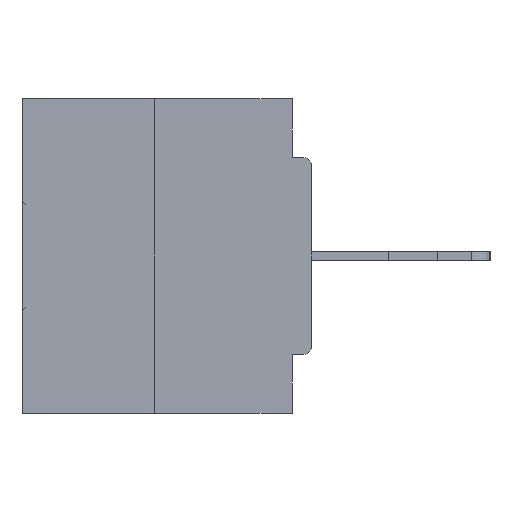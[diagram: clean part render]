
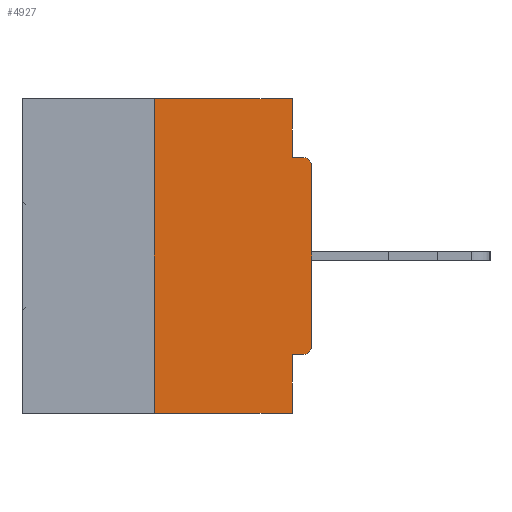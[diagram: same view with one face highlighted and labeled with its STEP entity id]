
A CAD part, left-side view. The second image highlights one B-rep face of the part: STEP entity #4927.
In plain terms, the highlighted planar face has unit normal (-1, 0, 0).
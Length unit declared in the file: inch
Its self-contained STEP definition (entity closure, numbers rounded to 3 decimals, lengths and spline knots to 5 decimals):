
#531 = CARTESIAN_POINT ( 'NONE',  ( 0., 0.031, -0.0935 ) ) ;
#1636 = DIRECTION ( 'NONE',  ( 0., 0., -1. ) ) ;
#2308 = LINE ( 'NONE', #13980, #9226 ) ;
#3226 = CIRCLE ( 'NONE', #31526, 0.015 ) ;
#3934 = EDGE_LOOP ( 'NONE', ( #4821, #33900, #36060, #4055, #22363, #35218, #20865, #37956, #14118, #7076 ) ) ;
#4055 = ORIENTED_EDGE ( 'NONE', *, *, #14420, .F. ) ;
#4821 = ORIENTED_EDGE ( 'NONE', *, *, #16176, .F. ) ;
#4909 = CARTESIAN_POINT ( 'NONE',  ( 0., 0.015, -0.4065 ) ) ;
#4925 = EDGE_CURVE ( 'NONE', #9672, #5532, #18148, .T. ) ;
#4927 = ADVANCED_FACE ( 'NONE', ( #14005 ), #31725, .F. ) ;
#5532 = VERTEX_POINT ( 'NONE', #37963 ) ;
#5896 = DIRECTION ( 'NONE',  ( 0., 1., 0. ) ) ;
#6661 = CARTESIAN_POINT ( 'NONE',  ( 0., 0.031, 0. ) ) ;
#6985 = LINE ( 'NONE', #9278, #9764 ) ;
#7076 = ORIENTED_EDGE ( 'NONE', *, *, #26326, .F. ) ;
#7156 = CARTESIAN_POINT ( 'NONE',  ( 0., 0.031, 0. ) ) ;
#7387 = CIRCLE ( 'NONE', #19720, 0.015 ) ;
#7488 = LINE ( 'NONE', #26544, #23994 ) ;
#7517 = CARTESIAN_POINT ( 'NONE',  ( 0., 0.031, -0.5 ) ) ;
#7746 = CARTESIAN_POINT ( 'NONE',  ( 0., 0.46, 0. ) ) ;
#8172 = VECTOR ( 'NONE', #13824, 39.37008 ) ;
#9226 = VECTOR ( 'NONE', #13871, 39.37008 ) ;
#9278 = CARTESIAN_POINT ( 'NONE',  ( 0., 0., -0.0935 ) ) ;
#9461 = CARTESIAN_POINT ( 'NONE',  ( 0., 0.015, -0.0935 ) ) ;
#9672 = VERTEX_POINT ( 'NONE', #28063 ) ;
#9764 = VECTOR ( 'NONE', #35614, 39.37008 ) ;
#10068 = CARTESIAN_POINT ( 'NONE',  ( 0., 0.25, -0.5 ) ) ;
#10980 = VERTEX_POINT ( 'NONE', #7517 ) ;
#11596 = EDGE_CURVE ( 'NONE', #27751, #10980, #27896, .T. ) ;
#11610 = VERTEX_POINT ( 'NONE', #30232 ) ;
#13336 = CARTESIAN_POINT ( 'NONE',  ( 0., 0.031, -0.5 ) ) ;
#13824 = DIRECTION ( 'NONE',  ( 0., -1., 0. ) ) ;
#13871 = DIRECTION ( 'NONE',  ( 0., 0., 1. ) ) ;
#13980 = CARTESIAN_POINT ( 'NONE',  ( 0., 0.25, 0. ) ) ;
#14005 = FACE_OUTER_BOUND ( 'NONE', #3934, .T. ) ;
#14103 = LINE ( 'NONE', #7156, #20996 ) ;
#14118 = ORIENTED_EDGE ( 'NONE', *, *, #14304, .F. ) ;
#14121 = DIRECTION ( 'NONE',  ( 1., 0., 0. ) ) ;
#14304 = EDGE_CURVE ( 'NONE', #31875, #31594, #6985, .T. ) ;
#14420 = EDGE_CURVE ( 'NONE', #11610, #10980, #31343, .T. ) ;
#15109 = EDGE_CURVE ( 'NONE', #17401, #9672, #7387, .T. ) ;
#15179 = DIRECTION ( 'NONE',  ( -1., 0., 0. ) ) ;
#15277 = EDGE_CURVE ( 'NONE', #27751, #17483, #2308, .T. ) ;
#15496 = CARTESIAN_POINT ( 'NONE',  ( 0., 0.46, -0.5 ) ) ;
#15572 = EDGE_CURVE ( 'NONE', #5532, #31594, #3226, .T. ) ;
#16176 = EDGE_CURVE ( 'NONE', #17483, #32365, #19649, .T. ) ;
#17401 = VERTEX_POINT ( 'NONE', #4909 ) ;
#17483 = VERTEX_POINT ( 'NONE', #27955 ) ;
#18002 = CARTESIAN_POINT ( 'NONE',  ( 0., 0.015, -0.3915 ) ) ;
#18148 = LINE ( 'NONE', #37544, #33782 ) ;
#18956 = DIRECTION ( 'NONE',  ( 0., 0., -1. ) ) ;
#19649 = LINE ( 'NONE', #22264, #8172 ) ;
#19720 = AXIS2_PLACEMENT_3D ( 'NONE', #18002, #15179, #29422 ) ;
#19989 = EDGE_CURVE ( 'NONE', #17401, #11610, #7488, .T. ) ;
#20865 = ORIENTED_EDGE ( 'NONE', *, *, #4925, .T. ) ;
#20996 = VECTOR ( 'NONE', #18956, 39.37008 ) ;
#22264 = CARTESIAN_POINT ( 'NONE',  ( 0., 0.46, 0. ) ) ;
#22363 = ORIENTED_EDGE ( 'NONE', *, *, #19989, .F. ) ;
#23994 = VECTOR ( 'NONE', #5896, 39.37008 ) ;
#24703 = VECTOR ( 'NONE', #36078, 39.37008 ) ;
#25603 = CARTESIAN_POINT ( 'NONE',  ( 0., 0.015, -0.1085 ) ) ;
#25804 = DIRECTION ( 'NONE',  ( 0., 0., 1. ) ) ;
#25979 = DIRECTION ( 'NONE',  ( 0., 0., -1. ) ) ;
#26326 = EDGE_CURVE ( 'NONE', #32365, #31875, #14103, .T. ) ;
#26544 = CARTESIAN_POINT ( 'NONE',  ( 0., 0., -0.4065 ) ) ;
#27751 = VERTEX_POINT ( 'NONE', #10068 ) ;
#27896 = LINE ( 'NONE', #15496, #24703 ) ;
#27955 = CARTESIAN_POINT ( 'NONE',  ( 0., 0.25, 0. ) ) ;
#28063 = CARTESIAN_POINT ( 'NONE',  ( 0., 0., -0.3915 ) ) ;
#29422 = DIRECTION ( 'NONE',  ( 0., 0., -1. ) ) ;
#30232 = CARTESIAN_POINT ( 'NONE',  ( 0., 0.031, -0.4065 ) ) ;
#31108 = AXIS2_PLACEMENT_3D ( 'NONE', #7746, #14121, #34707 ) ;
#31343 = LINE ( 'NONE', #13336, #33632 ) ;
#31526 = AXIS2_PLACEMENT_3D ( 'NONE', #25603, #34762, #25979 ) ;
#31594 = VERTEX_POINT ( 'NONE', #9461 ) ;
#31725 = PLANE ( 'NONE',  #31108 ) ;
#31875 = VERTEX_POINT ( 'NONE', #531 ) ;
#32365 = VERTEX_POINT ( 'NONE', #6661 ) ;
#33632 = VECTOR ( 'NONE', #1636, 39.37008 ) ;
#33782 = VECTOR ( 'NONE', #25804, 39.37008 ) ;
#33900 = ORIENTED_EDGE ( 'NONE', *, *, #15277, .F. ) ;
#34707 = DIRECTION ( 'NONE',  ( 0., 0., -1. ) ) ;
#34762 = DIRECTION ( 'NONE',  ( -1., 0., 0. ) ) ;
#35218 = ORIENTED_EDGE ( 'NONE', *, *, #15109, .T. ) ;
#35614 = DIRECTION ( 'NONE',  ( 0., -1., 0. ) ) ;
#36060 = ORIENTED_EDGE ( 'NONE', *, *, #11596, .T. ) ;
#36078 = DIRECTION ( 'NONE',  ( 0., -1., 0. ) ) ;
#37544 = CARTESIAN_POINT ( 'NONE',  ( 0., 0., 0. ) ) ;
#37956 = ORIENTED_EDGE ( 'NONE', *, *, #15572, .T. ) ;
#37963 = CARTESIAN_POINT ( 'NONE',  ( 0., 0., -0.1085 ) ) ;
